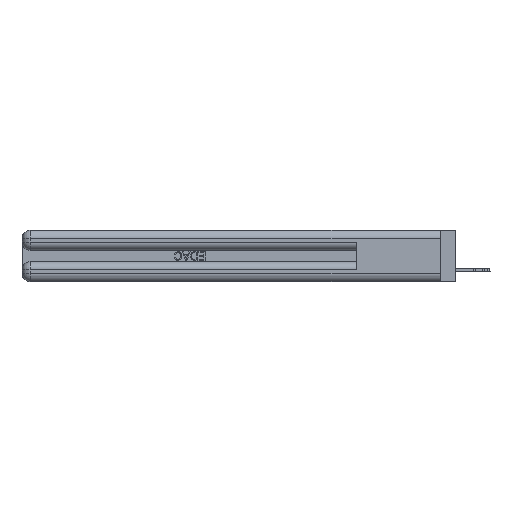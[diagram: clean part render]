
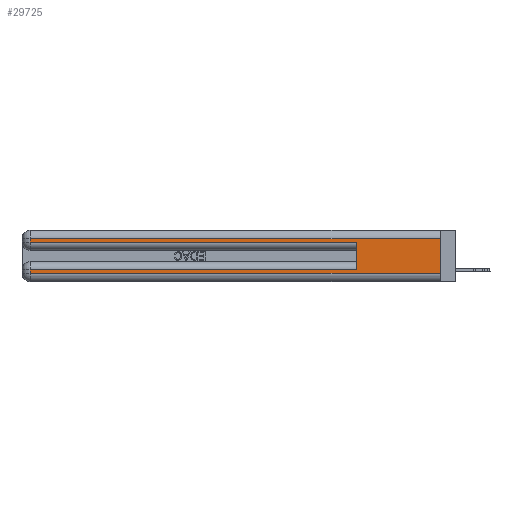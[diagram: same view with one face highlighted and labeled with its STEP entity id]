
A CAD part, left-side view. The second image highlights one B-rep face of the part: STEP entity #29725.
In plain terms, the highlighted planar face has unit normal (-1, 0, 0).
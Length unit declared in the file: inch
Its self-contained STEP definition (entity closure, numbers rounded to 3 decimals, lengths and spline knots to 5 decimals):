
#119 = EDGE_CURVE ( 'NONE', #3952, #35273, #35163, .T. ) ;
#272 = CARTESIAN_POINT ( 'NONE',  ( 0., 0.6, 0.145 ) ) ;
#1101 = LINE ( 'NONE', #16063, #12361 ) ;
#1905 = VECTOR ( 'NONE', #8475, 39.37008 ) ;
#1924 = CARTESIAN_POINT ( 'NONE',  ( 0., 0., 0.37 ) ) ;
#3118 = LINE ( 'NONE', #1924, #9290 ) ;
#3123 = VERTEX_POINT ( 'NONE', #30723 ) ;
#3952 = VERTEX_POINT ( 'NONE', #33682 ) ;
#4689 = CARTESIAN_POINT ( 'NONE',  ( 0., 0., 0.06 ) ) ;
#5469 = CARTESIAN_POINT ( 'NONE',  ( 0., 0., 0.31 ) ) ;
#5750 = DIRECTION ( 'NONE',  ( 1., 0., 0. ) ) ;
#6733 = CARTESIAN_POINT ( 'NONE',  ( 0., 0.6, 0.085 ) ) ;
#7105 = VECTOR ( 'NONE', #14494, 39.37008 ) ;
#7351 = VERTEX_POINT ( 'NONE', #17976 ) ;
#7474 = ORIENTED_EDGE ( 'NONE', *, *, #119, .T. ) ;
#8475 = DIRECTION ( 'NONE',  ( 0., -1., 0. ) ) ;
#8913 = DIRECTION ( 'NONE',  ( 0., 0., -1. ) ) ;
#9001 = VECTOR ( 'NONE', #8913, 39.37008 ) ;
#9290 = VECTOR ( 'NONE', #40487, 39.37008 ) ;
#9464 = DIRECTION ( 'NONE',  ( 0., 1., 0. ) ) ;
#9477 = LINE ( 'NONE', #21764, #9001 ) ;
#9557 = LINE ( 'NONE', #16096, #16683 ) ;
#9720 = EDGE_CURVE ( 'NONE', #22443, #37448, #1101, .T. ) ;
#9842 = CARTESIAN_POINT ( 'NONE',  ( 0., 0., 0.085 ) ) ;
#11659 = CARTESIAN_POINT ( 'NONE',  ( 0., 0., 0.285 ) ) ;
#12361 = VECTOR ( 'NONE', #26061, 39.37008 ) ;
#12455 = PLANE ( 'NONE',  #24978 ) ;
#12719 = EDGE_CURVE ( 'NONE', #22443, #35273, #3118, .T. ) ;
#13117 = DIRECTION ( 'NONE',  ( 0., 0., 1. ) ) ;
#13138 = EDGE_CURVE ( 'NONE', #37448, #14290, #9477, .T. ) ;
#13602 = VERTEX_POINT ( 'NONE', #6733 ) ;
#14290 = VERTEX_POINT ( 'NONE', #21338 ) ;
#14494 = DIRECTION ( 'NONE',  ( 0., -1., 0. ) ) ;
#14993 = EDGE_CURVE ( 'NONE', #13602, #7351, #38513, .T. ) ;
#15888 = LINE ( 'NONE', #11659, #7105 ) ;
#16063 = CARTESIAN_POINT ( 'NONE',  ( 0., 0., 0.31 ) ) ;
#16096 = CARTESIAN_POINT ( 'NONE',  ( 0., 2.94, 0.37 ) ) ;
#16683 = VECTOR ( 'NONE', #19123, 39.37008 ) ;
#17976 = CARTESIAN_POINT ( 'NONE',  ( 0., 2.94, 0.085 ) ) ;
#18378 = ORIENTED_EDGE ( 'NONE', *, *, #12719, .F. ) ;
#18578 = EDGE_CURVE ( 'NONE', #7351, #3952, #9557, .T. ) ;
#18794 = DIRECTION ( 'NONE',  ( 0., 0., -1. ) ) ;
#19123 = DIRECTION ( 'NONE',  ( 0., 0., -1. ) ) ;
#21338 = CARTESIAN_POINT ( 'NONE',  ( 0., 2.94, 0.285 ) ) ;
#21764 = CARTESIAN_POINT ( 'NONE',  ( 0., 2.94, 0.37 ) ) ;
#22443 = VERTEX_POINT ( 'NONE', #5469 ) ;
#22941 = ORIENTED_EDGE ( 'NONE', *, *, #14993, .T. ) ;
#23979 = ORIENTED_EDGE ( 'NONE', *, *, #37128, .T. ) ;
#24978 = AXIS2_PLACEMENT_3D ( 'NONE', #38515, #5750, #18794 ) ;
#25031 = EDGE_LOOP ( 'NONE', ( #18378, #41551, #25816, #23979, #35903, #22941, #31475, #7474 ) ) ;
#25169 = LINE ( 'NONE', #272, #31274 ) ;
#25816 = ORIENTED_EDGE ( 'NONE', *, *, #13138, .T. ) ;
#26061 = DIRECTION ( 'NONE',  ( 0., 1., 0. ) ) ;
#26671 = EDGE_CURVE ( 'NONE', #13602, #3123, #25169, .T. ) ;
#29258 = CARTESIAN_POINT ( 'NONE',  ( 0., 2.94, 0.31 ) ) ;
#29725 = ADVANCED_FACE ( 'NONE', ( #33814 ), #12455, .F. ) ;
#30723 = CARTESIAN_POINT ( 'NONE',  ( 0., 0.6, 0.285 ) ) ;
#31274 = VECTOR ( 'NONE', #13117, 39.37008 ) ;
#31475 = ORIENTED_EDGE ( 'NONE', *, *, #18578, .T. ) ;
#33330 = VECTOR ( 'NONE', #9464, 39.37008 ) ;
#33682 = CARTESIAN_POINT ( 'NONE',  ( 0., 2.94, 0.06 ) ) ;
#33814 = FACE_OUTER_BOUND ( 'NONE', #25031, .T. ) ;
#35163 = LINE ( 'NONE', #4689, #1905 ) ;
#35273 = VERTEX_POINT ( 'NONE', #37481 ) ;
#35903 = ORIENTED_EDGE ( 'NONE', *, *, #26671, .F. ) ;
#37128 = EDGE_CURVE ( 'NONE', #14290, #3123, #15888, .T. ) ;
#37448 = VERTEX_POINT ( 'NONE', #29258 ) ;
#37481 = CARTESIAN_POINT ( 'NONE',  ( 0., 0., 0.06 ) ) ;
#38513 = LINE ( 'NONE', #9842, #33330 ) ;
#38515 = CARTESIAN_POINT ( 'NONE',  ( 0., 0., 0.37 ) ) ;
#40487 = DIRECTION ( 'NONE',  ( 0., 0., -1. ) ) ;
#41551 = ORIENTED_EDGE ( 'NONE', *, *, #9720, .T. ) ;
